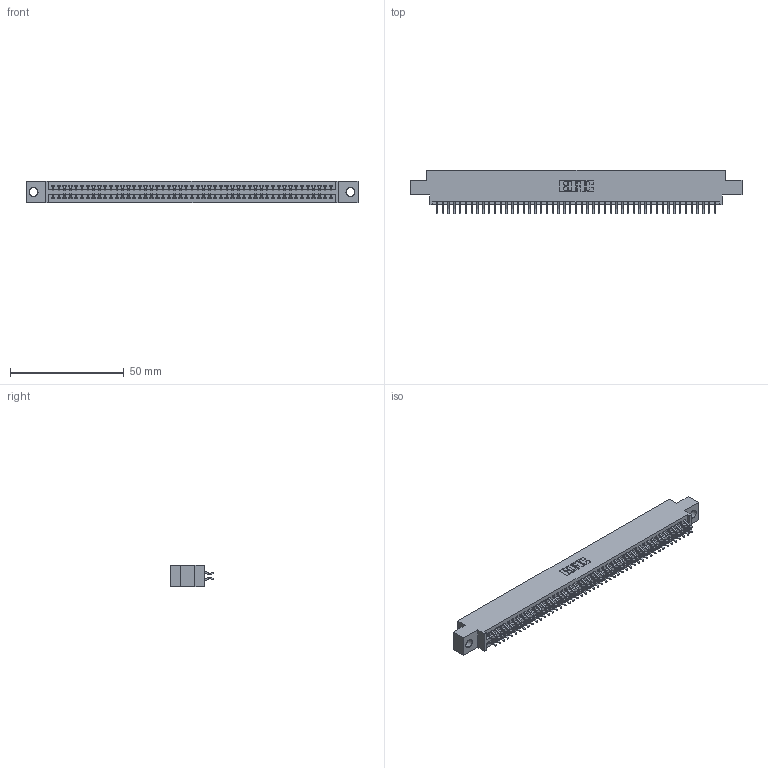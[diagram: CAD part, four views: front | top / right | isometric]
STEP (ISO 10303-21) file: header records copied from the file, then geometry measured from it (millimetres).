
FILE_DESCRIPTION (( 'STEP AP203' ), '1' );
FILE_NAME ('345-098-556-804.STEP', '2018-10-05T11:22:24', ( '' ), ( '' ), 'SwSTEP 2.0', 'SolidWorks 2016', '' );
FILE_SCHEMA (( 'CONFIG_CONTROL_DESIGN' ));
Length unit declared in the file: inch
Products named in the file (3): 345 Part_0.170 Offset - 0.156 Dia-TH; 345-098-556-804; 345-292-001_556 Tail
Assembly tree (99 placements, depth 2):
  345-098-556-804
    345 Part_0.170 Offset - 0.156 Dia-TH
    345-292-001_556 Tail  x98
Bounding box: 145.67 x 19.24 x 9.4 mm (x, y, z)
Volume: 14010.3 mm3; surface area: 20718 mm2
Topology: 99 solids, 99 shells, 5618 faces, 16719 edges, 11014 vertices
Faces by surface type: plane 3710, cylinder 1908
Entity records: 37859 total; most frequent: CARTESIAN_POINT 6356, ORIENTED_EDGE 6278, DIRECTION 5583, EDGE_CURVE 3139, VECTOR 2803, LINE 2803, VERTEX_POINT 2090, AXIS2_PLACEMENT_3D 1390
